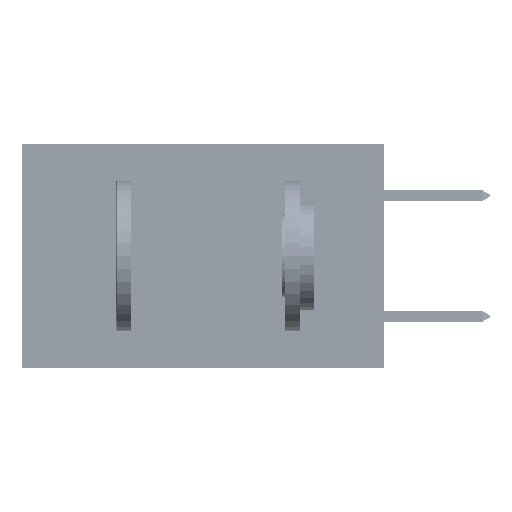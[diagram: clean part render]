
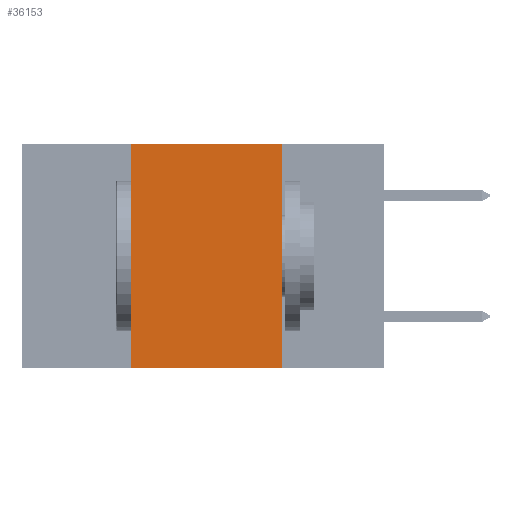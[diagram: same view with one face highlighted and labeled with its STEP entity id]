
A CAD part, left-side view. The second image highlights one B-rep face of the part: STEP entity #36153.
In plain terms, the highlighted planar face has unit normal (-1, 0, 0).
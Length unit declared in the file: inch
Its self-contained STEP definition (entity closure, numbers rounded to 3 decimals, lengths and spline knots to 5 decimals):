
#1213 = EDGE_CURVE ( 'NONE', #45200, #21364, #45156, .T. ) ;
#1624 = CARTESIAN_POINT ( 'NONE',  ( 0., 0.17, 0. ) ) ;
#2297 = ORIENTED_EDGE ( 'NONE', *, *, #18214, .F. ) ;
#3789 = VECTOR ( 'NONE', #34851, 39.37008 ) ;
#4549 = VECTOR ( 'NONE', #13299, 39.37008 ) ;
#5471 = VERTEX_POINT ( 'NONE', #17279 ) ;
#6674 = AXIS2_PLACEMENT_3D ( 'NONE', #20516, #24340, #28022 ) ;
#8441 = LINE ( 'NONE', #34392, #4549 ) ;
#9313 = LINE ( 'NONE', #31432, #14237 ) ;
#13011 = CARTESIAN_POINT ( 'NONE',  ( 0., 0.17, 0. ) ) ;
#13299 = DIRECTION ( 'NONE',  ( 0., -1., 0. ) ) ;
#14237 = VECTOR ( 'NONE', #41474, 39.37008 ) ;
#14833 = FACE_OUTER_BOUND ( 'NONE', #20378, .T. ) ;
#16740 = EDGE_CURVE ( 'NONE', #5471, #34574, #8441, .T. ) ;
#17279 = CARTESIAN_POINT ( 'NONE',  ( 0., 0.42, -0.37 ) ) ;
#18214 = EDGE_CURVE ( 'NONE', #21364, #34574, #41087, .T. ) ;
#19583 = ORIENTED_EDGE ( 'NONE', *, *, #1213, .F. ) ;
#20378 = EDGE_LOOP ( 'NONE', ( #2297, #19583, #32442, #38877 ) ) ;
#20516 = CARTESIAN_POINT ( 'NONE',  ( 0., 0.6, 0. ) ) ;
#20702 = CARTESIAN_POINT ( 'NONE',  ( 0., 0.6, 0. ) ) ;
#21364 = VERTEX_POINT ( 'NONE', #1624 ) ;
#24340 = DIRECTION ( 'NONE',  ( 1., 0., 0. ) ) ;
#27295 = DIRECTION ( 'NONE',  ( 0., 0., -1. ) ) ;
#28022 = DIRECTION ( 'NONE',  ( 0., 0., -1. ) ) ;
#31109 = CARTESIAN_POINT ( 'NONE',  ( 0., 0.17, -0.37 ) ) ;
#31432 = CARTESIAN_POINT ( 'NONE',  ( 0., 0.42, 0. ) ) ;
#32442 = ORIENTED_EDGE ( 'NONE', *, *, #45385, .F. ) ;
#33905 = VECTOR ( 'NONE', #27295, 39.37008 ) ;
#34392 = CARTESIAN_POINT ( 'NONE',  ( 0., 0.6, -0.37 ) ) ;
#34574 = VERTEX_POINT ( 'NONE', #31109 ) ;
#34646 = PLANE ( 'NONE',  #6674 ) ;
#34851 = DIRECTION ( 'NONE',  ( 0., -1., 0. ) ) ;
#36153 = ADVANCED_FACE ( 'NONE', ( #14833 ), #34646, .F. ) ;
#38877 = ORIENTED_EDGE ( 'NONE', *, *, #16740, .T. ) ;
#41087 = LINE ( 'NONE', #13011, #33905 ) ;
#41474 = DIRECTION ( 'NONE',  ( 0., 0., 1. ) ) ;
#44408 = CARTESIAN_POINT ( 'NONE',  ( 0., 0.42, 0. ) ) ;
#45156 = LINE ( 'NONE', #20702, #3789 ) ;
#45200 = VERTEX_POINT ( 'NONE', #44408 ) ;
#45385 = EDGE_CURVE ( 'NONE', #5471, #45200, #9313, .T. ) ;
